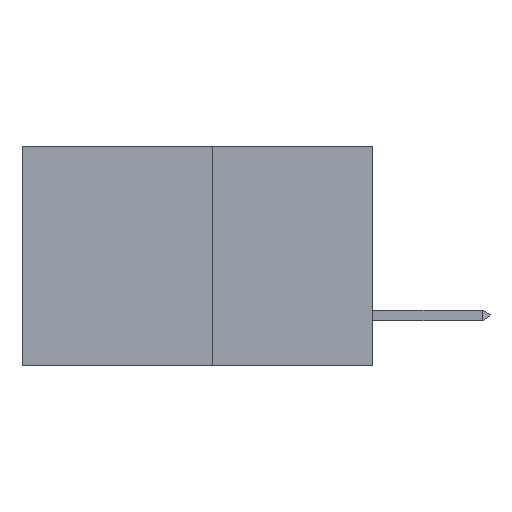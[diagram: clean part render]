
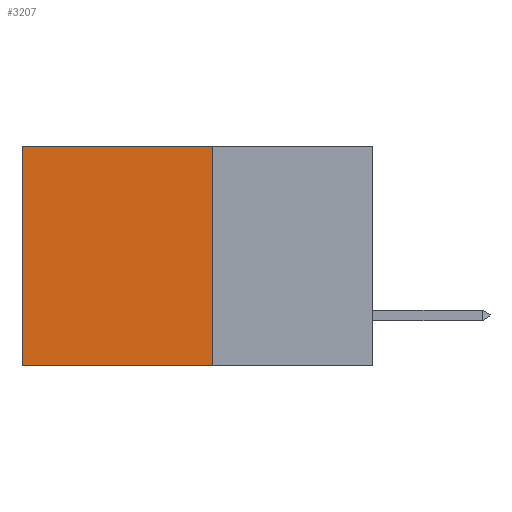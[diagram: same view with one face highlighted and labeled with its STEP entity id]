
A CAD part, left-side view. The second image highlights one B-rep face of the part: STEP entity #3207.
In plain terms, the highlighted planar face has unit normal (-1, 0, 0).
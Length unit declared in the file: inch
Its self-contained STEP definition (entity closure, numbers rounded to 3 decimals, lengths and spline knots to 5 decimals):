
#153 = CARTESIAN_POINT ( 'NONE',  ( 0.277, 0.59, -0.37 ) ) ;
#253 = VECTOR ( 'NONE', #2340, 39.37008 ) ;
#866 = ORIENTED_EDGE ( 'NONE', *, *, #17427, .T. ) ;
#998 = DIRECTION ( 'NONE',  ( 0., 0., -1. ) ) ;
#1190 = CARTESIAN_POINT ( 'NONE',  ( 0.277, 0.59, -0.37 ) ) ;
#1241 = LINE ( 'NONE', #23306, #10266 ) ;
#1417 = ORIENTED_EDGE ( 'NONE', *, *, #6823, .F. ) ;
#1573 = VERTEX_POINT ( 'NONE', #11672 ) ;
#1694 = DIRECTION ( 'NONE',  ( 0., 1., 0. ) ) ;
#2340 = DIRECTION ( 'NONE',  ( 0., 1., 0. ) ) ;
#3207 = ADVANCED_FACE ( 'NONE', ( #22883 ), #10775, .F. ) ;
#5322 = LINE ( 'NONE', #22444, #19125 ) ;
#5568 = VERTEX_POINT ( 'NONE', #11193 ) ;
#6593 = EDGE_CURVE ( 'NONE', #5568, #20020, #7292, .T. ) ;
#6823 = EDGE_CURVE ( 'NONE', #1573, #13855, #5322, .T. ) ;
#7292 = LINE ( 'NONE', #1190, #15763 ) ;
#9788 = DIRECTION ( 'NONE',  ( 0., 0., -1. ) ) ;
#9888 = DIRECTION ( 'NONE',  ( 1., 0., 0. ) ) ;
#10266 = VECTOR ( 'NONE', #1694, 39.37008 ) ;
#10775 = PLANE ( 'NONE',  #19834 ) ;
#10822 = CARTESIAN_POINT ( 'NONE',  ( 0.277, 0.27, -0.37 ) ) ;
#11193 = CARTESIAN_POINT ( 'NONE',  ( 0.277, 0.59, 0. ) ) ;
#11672 = CARTESIAN_POINT ( 'NONE',  ( 0.277, 0.27, 0. ) ) ;
#13855 = VERTEX_POINT ( 'NONE', #17919 ) ;
#14853 = ORIENTED_EDGE ( 'NONE', *, *, #6593, .T. ) ;
#15216 = LINE ( 'NONE', #18510, #253 ) ;
#15699 = ORIENTED_EDGE ( 'NONE', *, *, #18988, .F. ) ;
#15763 = VECTOR ( 'NONE', #998, 39.37008 ) ;
#17427 = EDGE_CURVE ( 'NONE', #1573, #5568, #1241, .T. ) ;
#17919 = CARTESIAN_POINT ( 'NONE',  ( 0.277, 0.27, -0.37 ) ) ;
#18013 = DIRECTION ( 'NONE',  ( 0., 0., -1. ) ) ;
#18230 = EDGE_LOOP ( 'NONE', ( #14853, #15699, #1417, #866 ) ) ;
#18510 = CARTESIAN_POINT ( 'NONE',  ( 0.277, 0.27, -0.37 ) ) ;
#18988 = EDGE_CURVE ( 'NONE', #13855, #20020, #15216, .T. ) ;
#19125 = VECTOR ( 'NONE', #18013, 39.37008 ) ;
#19834 = AXIS2_PLACEMENT_3D ( 'NONE', #10822, #9888, #9788 ) ;
#20020 = VERTEX_POINT ( 'NONE', #153 ) ;
#22444 = CARTESIAN_POINT ( 'NONE',  ( 0.277, 0.27, -0.37 ) ) ;
#22883 = FACE_OUTER_BOUND ( 'NONE', #18230, .T. ) ;
#23306 = CARTESIAN_POINT ( 'NONE',  ( 0.277, 0.27, 0. ) ) ;
